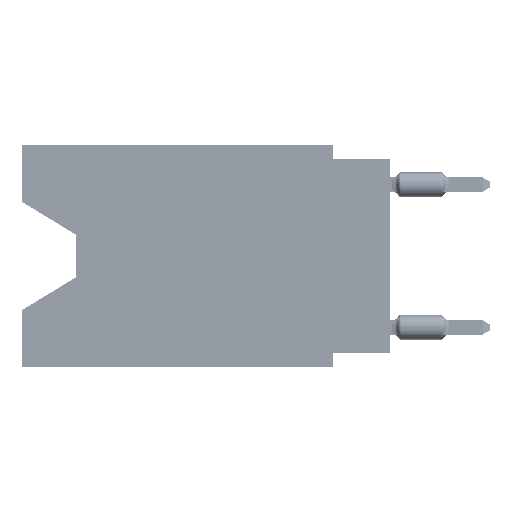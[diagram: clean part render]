
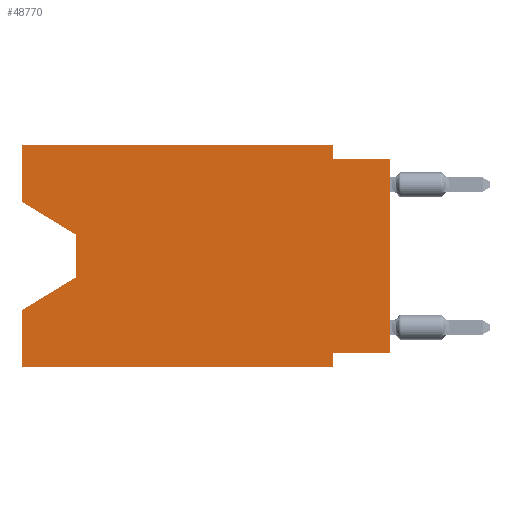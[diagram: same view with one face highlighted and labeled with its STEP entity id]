
A CAD part, left-side view. The second image highlights one B-rep face of the part: STEP entity #48770.
In plain terms, the highlighted planar face has unit normal (-1, 0, 0).
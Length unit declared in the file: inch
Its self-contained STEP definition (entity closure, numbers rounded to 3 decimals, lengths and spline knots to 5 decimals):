
#491 = ORIENTED_EDGE ( 'NONE', *, *, #15521, .T. ) ;
#1272 = CARTESIAN_POINT ( 'NONE',  ( 0., 0., -0.365 ) ) ;
#1378 = CARTESIAN_POINT ( 'NONE',  ( 0., 0., 0. ) ) ;
#2271 = CARTESIAN_POINT ( 'NONE',  ( 0., 0.645, -0.10025 ) ) ;
#2693 = VERTEX_POINT ( 'NONE', #23991 ) ;
#3446 = CARTESIAN_POINT ( 'NONE',  ( 0., 0.55, -0.158 ) ) ;
#3863 = ORIENTED_EDGE ( 'NONE', *, *, #22986, .F. ) ;
#4157 = VECTOR ( 'NONE', #24867, 39.37008 ) ;
#4220 = CARTESIAN_POINT ( 'NONE',  ( 0., 0.645, 0. ) ) ;
#4489 = EDGE_CURVE ( 'NONE', #8692, #34043, #49778, .T. ) ;
#7193 = CARTESIAN_POINT ( 'NONE',  ( 0., 0.55, -0.232 ) ) ;
#7797 = CARTESIAN_POINT ( 'NONE',  ( 0., 0.1, -0.025 ) ) ;
#8202 = CARTESIAN_POINT ( 'NONE',  ( 0., 0.645, -0.39 ) ) ;
#8271 = DIRECTION ( 'NONE',  ( 0., 0., -1. ) ) ;
#8416 = DIRECTION ( 'NONE',  ( 0., 0., 1. ) ) ;
#8692 = VERTEX_POINT ( 'NONE', #1272 ) ;
#9328 = VERTEX_POINT ( 'NONE', #8202 ) ;
#9481 = VECTOR ( 'NONE', #27580, 39.37008 ) ;
#11891 = CARTESIAN_POINT ( 'NONE',  ( 0., 0.1, 0. ) ) ;
#12263 = ORIENTED_EDGE ( 'NONE', *, *, #65582, .F. ) ;
#13978 = CARTESIAN_POINT ( 'NONE',  ( 0., 0.645, 0. ) ) ;
#14043 = CARTESIAN_POINT ( 'NONE',  ( 0., 0.1, -0.39 ) ) ;
#15521 = EDGE_CURVE ( 'NONE', #62178, #26670, #64954, .T. ) ;
#15678 = CARTESIAN_POINT ( 'NONE',  ( 0., 0., -0.365 ) ) ;
#16447 = CARTESIAN_POINT ( 'NONE',  ( 0., 0., -0.025 ) ) ;
#17838 = CARTESIAN_POINT ( 'NONE',  ( 0., 0.1, 0. ) ) ;
#19735 = ORIENTED_EDGE ( 'NONE', *, *, #26415, .T. ) ;
#20481 = DIRECTION ( 'NONE',  ( 0., 0., -1. ) ) ;
#20990 = EDGE_CURVE ( 'NONE', #2693, #62178, #53037, .T. ) ;
#22092 = DIRECTION ( 'NONE',  ( 1., 0., 0. ) ) ;
#22986 = EDGE_CURVE ( 'NONE', #72014, #37055, #23979, .T. ) ;
#23113 = LINE ( 'NONE', #51661, #9481 ) ;
#23640 = VECTOR ( 'NONE', #40564, 39.37008 ) ;
#23893 = ORIENTED_EDGE ( 'NONE', *, *, #42373, .T. ) ;
#23979 = LINE ( 'NONE', #69186, #56418 ) ;
#23991 = CARTESIAN_POINT ( 'NONE',  ( 0., 0.645, -0.10025 ) ) ;
#24119 = VERTEX_POINT ( 'NONE', #47287 ) ;
#24867 = DIRECTION ( 'NONE',  ( 0., -0.855, -0.519 ) ) ;
#25333 = VECTOR ( 'NONE', #38296, 39.37008 ) ;
#26415 = EDGE_CURVE ( 'NONE', #8692, #24119, #57329, .T. ) ;
#26670 = VERTEX_POINT ( 'NONE', #71384 ) ;
#27580 = DIRECTION ( 'NONE',  ( 0., -1., 0. ) ) ;
#28568 = ORIENTED_EDGE ( 'NONE', *, *, #4489, .F. ) ;
#28953 = LINE ( 'NONE', #11891, #53038 ) ;
#29002 = DIRECTION ( 'NONE',  ( 0., 0., 1. ) ) ;
#29427 = EDGE_CURVE ( 'NONE', #37055, #61884, #28953, .T. ) ;
#32022 = VECTOR ( 'NONE', #20481, 39.37008 ) ;
#33707 = ORIENTED_EDGE ( 'NONE', *, *, #55801, .F. ) ;
#34043 = VERTEX_POINT ( 'NONE', #52115 ) ;
#36150 = AXIS2_PLACEMENT_3D ( 'NONE', #66952, #22092, #44706 ) ;
#36453 = VERTEX_POINT ( 'NONE', #60314 ) ;
#37055 = VERTEX_POINT ( 'NONE', #17838 ) ;
#38296 = DIRECTION ( 'NONE',  ( 0., 1., 0. ) ) ;
#39057 = DIRECTION ( 'NONE',  ( 0., -1., 0. ) ) ;
#39330 = DIRECTION ( 'NONE',  ( 0., 0., -1. ) ) ;
#40283 = DIRECTION ( 'NONE',  ( 0., 0., 1. ) ) ;
#40564 = DIRECTION ( 'NONE',  ( 0., 0.855, -0.519 ) ) ;
#41655 = LINE ( 'NONE', #7193, #23640 ) ;
#42373 = EDGE_CURVE ( 'NONE', #9328, #58646, #23113, .T. ) ;
#42649 = EDGE_CURVE ( 'NONE', #34043, #58646, #54560, .T. ) ;
#43471 = VECTOR ( 'NONE', #8271, 39.37008 ) ;
#44340 = PLANE ( 'NONE',  #36150 ) ;
#44706 = DIRECTION ( 'NONE',  ( 0., 0., -1. ) ) ;
#45426 = EDGE_LOOP ( 'NONE', ( #66719, #491, #57631, #68829, #23893, #51104, #28568, #19735, #12263, #46666, #3863, #33707 ) ) ;
#45697 = LINE ( 'NONE', #67913, #58610 ) ;
#46666 = ORIENTED_EDGE ( 'NONE', *, *, #29427, .F. ) ;
#47287 = CARTESIAN_POINT ( 'NONE',  ( 0., 0., -0.025 ) ) ;
#47480 = EDGE_CURVE ( 'NONE', #9328, #36453, #53633, .T. ) ;
#48280 = CARTESIAN_POINT ( 'NONE',  ( 0., 0.1, -0.39 ) ) ;
#48770 = ADVANCED_FACE ( 'NONE', ( #50991 ), #44340, .F. ) ;
#49778 = LINE ( 'NONE', #15678, #25333 ) ;
#50407 = VECTOR ( 'NONE', #40283, 39.37008 ) ;
#50991 = FACE_OUTER_BOUND ( 'NONE', #45426, .T. ) ;
#51104 = ORIENTED_EDGE ( 'NONE', *, *, #42649, .F. ) ;
#51661 = CARTESIAN_POINT ( 'NONE',  ( 0., 0.645, -0.39 ) ) ;
#51785 = DIRECTION ( 'NONE',  ( 0., -1., 0. ) ) ;
#52115 = CARTESIAN_POINT ( 'NONE',  ( 0., 0.1, -0.365 ) ) ;
#53037 = LINE ( 'NONE', #2271, #4157 ) ;
#53038 = VECTOR ( 'NONE', #39330, 39.37008 ) ;
#53633 = LINE ( 'NONE', #13978, #71584 ) ;
#54560 = LINE ( 'NONE', #48280, #32022 ) ;
#55801 = EDGE_CURVE ( 'NONE', #2693, #72014, #45697, .T. ) ;
#56418 = VECTOR ( 'NONE', #51785, 39.37008 ) ;
#57329 = LINE ( 'NONE', #1378, #50407 ) ;
#57631 = ORIENTED_EDGE ( 'NONE', *, *, #62614, .T. ) ;
#58610 = VECTOR ( 'NONE', #29002, 39.37008 ) ;
#58646 = VERTEX_POINT ( 'NONE', #14043 ) ;
#60314 = CARTESIAN_POINT ( 'NONE',  ( 0., 0.645, -0.28975 ) ) ;
#61829 = CARTESIAN_POINT ( 'NONE',  ( 0., 0.55, -0.158 ) ) ;
#61884 = VERTEX_POINT ( 'NONE', #7797 ) ;
#62178 = VERTEX_POINT ( 'NONE', #61829 ) ;
#62614 = EDGE_CURVE ( 'NONE', #26670, #36453, #41655, .T. ) ;
#62898 = VECTOR ( 'NONE', #39057, 39.37008 ) ;
#64954 = LINE ( 'NONE', #3446, #43471 ) ;
#65582 = EDGE_CURVE ( 'NONE', #61884, #24119, #67585, .T. ) ;
#66719 = ORIENTED_EDGE ( 'NONE', *, *, #20990, .T. ) ;
#66952 = CARTESIAN_POINT ( 'NONE',  ( 0., 0.645, 0. ) ) ;
#67585 = LINE ( 'NONE', #16447, #62898 ) ;
#67913 = CARTESIAN_POINT ( 'NONE',  ( 0., 0.645, 0. ) ) ;
#68829 = ORIENTED_EDGE ( 'NONE', *, *, #47480, .F. ) ;
#69186 = CARTESIAN_POINT ( 'NONE',  ( 0., 0.645, 0. ) ) ;
#71384 = CARTESIAN_POINT ( 'NONE',  ( 0., 0.55, -0.232 ) ) ;
#71584 = VECTOR ( 'NONE', #8416, 39.37008 ) ;
#72014 = VERTEX_POINT ( 'NONE', #4220 ) ;
